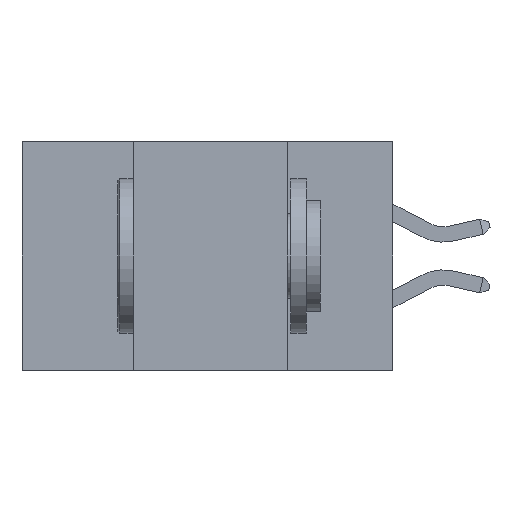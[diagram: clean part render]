
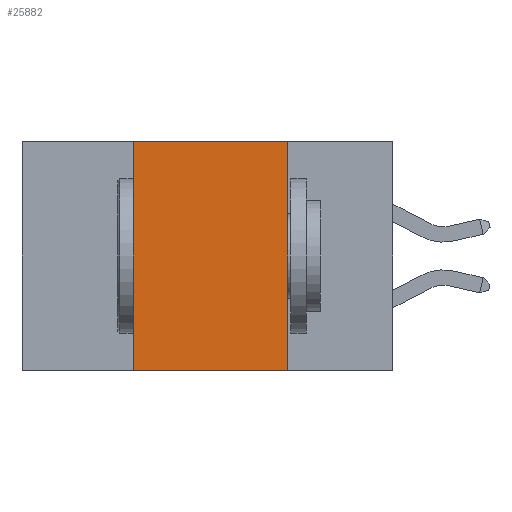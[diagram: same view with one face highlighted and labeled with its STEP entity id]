
A CAD part, left-side view. The second image highlights one B-rep face of the part: STEP entity #25882.
In plain terms, the highlighted planar face has unit normal (-1, 0, 0).
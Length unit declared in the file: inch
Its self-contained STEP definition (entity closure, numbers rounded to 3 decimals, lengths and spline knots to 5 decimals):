
#497 = ORIENTED_EDGE ( 'NONE', *, *, #16451, .T. ) ;
#1742 = CARTESIAN_POINT ( 'NONE',  ( 0., 0.6, -0.37 ) ) ;
#3556 = LINE ( 'NONE', #18692, #25473 ) ;
#4794 = FACE_OUTER_BOUND ( 'NONE', #21663, .T. ) ;
#5314 = CARTESIAN_POINT ( 'NONE',  ( 0., 0.42, 0. ) ) ;
#5356 = VECTOR ( 'NONE', #19548, 39.37008 ) ;
#6859 = LINE ( 'NONE', #24363, #12566 ) ;
#6925 = EDGE_CURVE ( 'NONE', #18259, #17896, #6859, .T. ) ;
#8204 = PLANE ( 'NONE',  #25366 ) ;
#9776 = CARTESIAN_POINT ( 'NONE',  ( 0., 0.17, 0. ) ) ;
#10298 = DIRECTION ( 'NONE',  ( 1., 0., 0. ) ) ;
#10328 = VERTEX_POINT ( 'NONE', #5314 ) ;
#11635 = ORIENTED_EDGE ( 'NONE', *, *, #6925, .F. ) ;
#12566 = VECTOR ( 'NONE', #26455, 39.37008 ) ;
#13203 = CARTESIAN_POINT ( 'NONE',  ( 0., 0.42, 0. ) ) ;
#14563 = DIRECTION ( 'NONE',  ( 0., -1., 0. ) ) ;
#14879 = LINE ( 'NONE', #1742, #25973 ) ;
#15669 = ORIENTED_EDGE ( 'NONE', *, *, #23102, .F. ) ;
#16335 = ORIENTED_EDGE ( 'NONE', *, *, #19215, .F. ) ;
#16451 = EDGE_CURVE ( 'NONE', #23860, #17896, #14879, .T. ) ;
#16797 = DIRECTION ( 'NONE',  ( 0., -1., 0. ) ) ;
#17896 = VERTEX_POINT ( 'NONE', #25465 ) ;
#18259 = VERTEX_POINT ( 'NONE', #9776 ) ;
#18692 = CARTESIAN_POINT ( 'NONE',  ( 0., 0.6, 0. ) ) ;
#19086 = CARTESIAN_POINT ( 'NONE',  ( 0., 0.42, -0.37 ) ) ;
#19215 = EDGE_CURVE ( 'NONE', #23860, #10328, #21606, .T. ) ;
#19548 = DIRECTION ( 'NONE',  ( 0., 0., 1. ) ) ;
#21606 = LINE ( 'NONE', #13203, #5356 ) ;
#21663 = EDGE_LOOP ( 'NONE', ( #11635, #15669, #16335, #497 ) ) ;
#22948 = CARTESIAN_POINT ( 'NONE',  ( 0., 0.6, 0. ) ) ;
#23102 = EDGE_CURVE ( 'NONE', #10328, #18259, #3556, .T. ) ;
#23860 = VERTEX_POINT ( 'NONE', #19086 ) ;
#24363 = CARTESIAN_POINT ( 'NONE',  ( 0., 0.17, 0. ) ) ;
#25055 = DIRECTION ( 'NONE',  ( 0., 0., -1. ) ) ;
#25366 = AXIS2_PLACEMENT_3D ( 'NONE', #22948, #10298, #25055 ) ;
#25465 = CARTESIAN_POINT ( 'NONE',  ( 0., 0.17, -0.37 ) ) ;
#25473 = VECTOR ( 'NONE', #14563, 39.37008 ) ;
#25882 = ADVANCED_FACE ( 'NONE', ( #4794 ), #8204, .F. ) ;
#25973 = VECTOR ( 'NONE', #16797, 39.37008 ) ;
#26455 = DIRECTION ( 'NONE',  ( 0., 0., -1. ) ) ;
